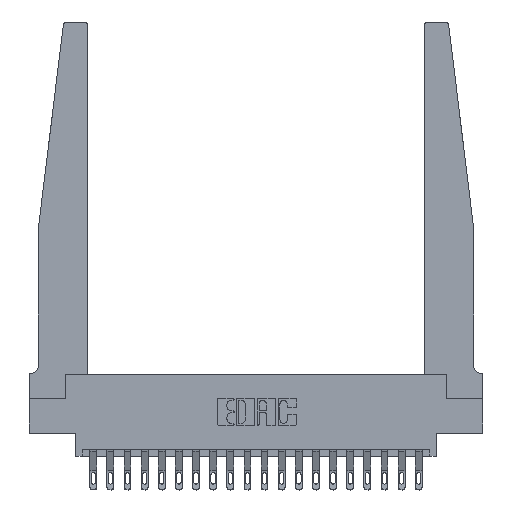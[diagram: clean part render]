
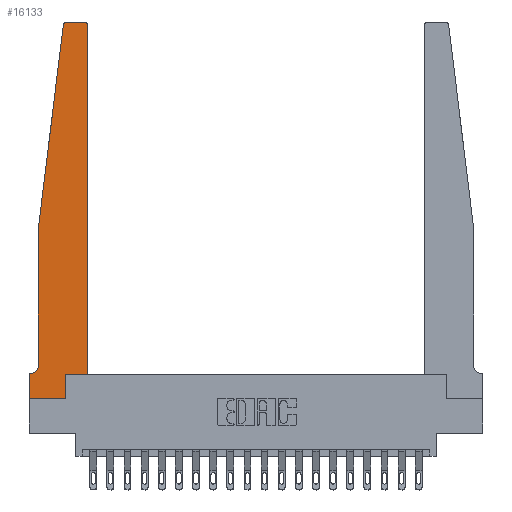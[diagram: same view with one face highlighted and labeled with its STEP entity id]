
A CAD part, top view. The second image highlights one B-rep face of the part: STEP entity #16133.
In plain terms, the highlighted planar face has unit normal (0, 0, 1).
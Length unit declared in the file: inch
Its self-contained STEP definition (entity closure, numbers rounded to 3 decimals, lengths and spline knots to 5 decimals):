
#439 = AXIS2_PLACEMENT_3D ( 'NONE', #8504, #13570, #7630 ) ;
#460 = ORIENTED_EDGE ( 'NONE', *, *, #15996, .T. ) ;
#556 = CARTESIAN_POINT ( 'NONE',  ( 0.425, 0.18, 0.37 ) ) ;
#888 = VERTEX_POINT ( 'NONE', #10330 ) ;
#1077 = DIRECTION ( 'NONE',  ( 0., -1., 0. ) ) ;
#1188 = CARTESIAN_POINT ( 'NONE',  ( 0., 0.1875, 0.37 ) ) ;
#1359 = VECTOR ( 'NONE', #13940, 39.37008 ) ;
#1505 = LINE ( 'NONE', #11701, #17941 ) ;
#1831 = PLANE ( 'NONE',  #439 ) ;
#1939 = DIRECTION ( 'NONE',  ( 1., 0., 0. ) ) ;
#1996 = VERTEX_POINT ( 'NONE', #8567 ) ;
#3223 = AXIS2_PLACEMENT_3D ( 'NONE', #15246, #12058, #15357 ) ;
#3746 = DIRECTION ( 'NONE',  ( 0., 1., 0. ) ) ;
#3941 = EDGE_CURVE ( 'NONE', #10184, #888, #16129, .T. ) ;
#4355 = ORIENTED_EDGE ( 'NONE', *, *, #3941, .T. ) ;
#4744 = LINE ( 'NONE', #11229, #5570 ) ;
#4805 = ORIENTED_EDGE ( 'NONE', *, *, #14903, .T. ) ;
#4994 = CARTESIAN_POINT ( 'NONE',  ( 0.2605, 0.18, 0.37 ) ) ;
#5111 = CARTESIAN_POINT ( 'NONE',  ( 0.065, 1.25, 0.37 ) ) ;
#5184 = EDGE_CURVE ( 'NONE', #16168, #1996, #13847, .T. ) ;
#5434 = CARTESIAN_POINT ( 'NONE',  ( 0.065, 1.25, 0.37 ) ) ;
#5570 = VECTOR ( 'NONE', #6393, 39.37008 ) ;
#5815 = VERTEX_POINT ( 'NONE', #21369 ) ;
#6218 = CARTESIAN_POINT ( 'NONE',  ( 0., 0., 0.37 ) ) ;
#6393 = DIRECTION ( 'NONE',  ( 1., 0., 0. ) ) ;
#6974 = ORIENTED_EDGE ( 'NONE', *, *, #12363, .T. ) ;
#7573 = DIRECTION ( 'NONE',  ( 1., 0., 0. ) ) ;
#7630 = DIRECTION ( 'NONE',  ( 1., 0., 0. ) ) ;
#7911 = LINE ( 'NONE', #16384, #16895 ) ;
#8035 = ORIENTED_EDGE ( 'NONE', *, *, #14879, .T. ) ;
#8504 = CARTESIAN_POINT ( 'NONE',  ( 0., 0.1875, 0.37 ) ) ;
#8559 = VERTEX_POINT ( 'NONE', #21633 ) ;
#8567 = CARTESIAN_POINT ( 'NONE',  ( 0.425, 2.72, 0.37 ) ) ;
#8787 = AXIS2_PLACEMENT_3D ( 'NONE', #10043, #13673, #1939 ) ;
#8823 = DIRECTION ( 'NONE',  ( 0., -1., 0. ) ) ;
#9060 = VECTOR ( 'NONE', #11697, 39.37008 ) ;
#9138 = ORIENTED_EDGE ( 'NONE', *, *, #15578, .T. ) ;
#9245 = VECTOR ( 'NONE', #8823, 39.37008 ) ;
#9516 = DIRECTION ( 'NONE',  ( 0., 0., 1. ) ) ;
#9721 = VERTEX_POINT ( 'NONE', #18452 ) ;
#9821 = LINE ( 'NONE', #5434, #9245 ) ;
#9900 = EDGE_CURVE ( 'NONE', #5815, #16168, #15599, .T. ) ;
#10043 = CARTESIAN_POINT ( 'NONE',  ( 0.27653, 2.72, 0.37 ) ) ;
#10184 = VERTEX_POINT ( 'NONE', #1188 ) ;
#10258 = VECTOR ( 'NONE', #3746, 39.37008 ) ;
#10330 = CARTESIAN_POINT ( 'NONE',  ( 0., 0., 0.37 ) ) ;
#10697 = ORIENTED_EDGE ( 'NONE', *, *, #9900, .T. ) ;
#11091 = ORIENTED_EDGE ( 'NONE', *, *, #12019, .T. ) ;
#11229 = CARTESIAN_POINT ( 'NONE',  ( 0., 0., 0.37 ) ) ;
#11468 = VERTEX_POINT ( 'NONE', #18428 ) ;
#11697 = DIRECTION ( 'NONE',  ( -0.122, -0.992, 0. ) ) ;
#11701 = CARTESIAN_POINT ( 'NONE',  ( 0.065, 0.1875, 0.37 ) ) ;
#11726 = VERTEX_POINT ( 'NONE', #16111 ) ;
#11958 = VECTOR ( 'NONE', #15109, 39.37008 ) ;
#12013 = ORIENTED_EDGE ( 'NONE', *, *, #19616, .T. ) ;
#12019 = EDGE_CURVE ( 'NONE', #18433, #13911, #15321, .T. ) ;
#12058 = DIRECTION ( 'NONE',  ( 0., 0., -1. ) ) ;
#12363 = EDGE_CURVE ( 'NONE', #888, #8559, #4744, .T. ) ;
#12481 = ORIENTED_EDGE ( 'NONE', *, *, #15734, .T. ) ;
#12696 = CARTESIAN_POINT ( 'NONE',  ( 0.24675, 2.72367, 0.37 ) ) ;
#13025 = CIRCLE ( 'NONE', #3223, 0.05 ) ;
#13570 = DIRECTION ( 'NONE',  ( 0., 0., 1. ) ) ;
#13673 = DIRECTION ( 'NONE',  ( 0., 0., 1. ) ) ;
#13790 = AXIS2_PLACEMENT_3D ( 'NONE', #17879, #9516, #7573 ) ;
#13847 = LINE ( 'NONE', #17475, #10258 ) ;
#13911 = VERTEX_POINT ( 'NONE', #14893 ) ;
#13940 = DIRECTION ( 'NONE',  ( 1., 0., 0. ) ) ;
#14299 = DIRECTION ( 'NONE',  ( -1., 0., 0. ) ) ;
#14879 = EDGE_CURVE ( 'NONE', #11468, #18433, #20018, .T. ) ;
#14893 = CARTESIAN_POINT ( 'NONE',  ( 0.065, 1.25, 0.37 ) ) ;
#14903 = EDGE_CURVE ( 'NONE', #8559, #5815, #18076, .T. ) ;
#14952 = DIRECTION ( 'NONE',  ( -1., 0., 0. ) ) ;
#15005 = FACE_OUTER_BOUND ( 'NONE', #18747, .T. ) ;
#15109 = DIRECTION ( 'NONE',  ( 0., 1., 0. ) ) ;
#15246 = CARTESIAN_POINT ( 'NONE',  ( 0.015, 0.2375, 0.37 ) ) ;
#15321 = LINE ( 'NONE', #5111, #9060 ) ;
#15357 = DIRECTION ( 'NONE',  ( -1., 0., 0. ) ) ;
#15578 = EDGE_CURVE ( 'NONE', #11726, #11468, #7911, .T. ) ;
#15599 = LINE ( 'NONE', #556, #1359 ) ;
#15734 = EDGE_CURVE ( 'NONE', #9721, #20816, #13025, .T. ) ;
#15996 = EDGE_CURVE ( 'NONE', #20816, #10184, #1505, .T. ) ;
#16111 = CARTESIAN_POINT ( 'NONE',  ( 0.395, 2.75, 0.37 ) ) ;
#16129 = LINE ( 'NONE', #6218, #20458 ) ;
#16133 = ADVANCED_FACE ( 'NONE', ( #15005 ), #1831, .T. ) ;
#16168 = VERTEX_POINT ( 'NONE', #18847 ) ;
#16384 = CARTESIAN_POINT ( 'NONE',  ( 0.25, 2.75, 0.37 ) ) ;
#16895 = VECTOR ( 'NONE', #14299, 39.37008 ) ;
#17260 = CARTESIAN_POINT ( 'NONE',  ( 0.015, 0.1875, 0.37 ) ) ;
#17316 = CIRCLE ( 'NONE', #13790, 0.03 ) ;
#17475 = CARTESIAN_POINT ( 'NONE',  ( 0.425, 0.18, 0.37 ) ) ;
#17685 = ORIENTED_EDGE ( 'NONE', *, *, #20126, .T. ) ;
#17879 = CARTESIAN_POINT ( 'NONE',  ( 0.395, 2.72, 0.37 ) ) ;
#17941 = VECTOR ( 'NONE', #14952, 39.37008 ) ;
#18076 = LINE ( 'NONE', #4994, #11958 ) ;
#18428 = CARTESIAN_POINT ( 'NONE',  ( 0.27653, 2.75, 0.37 ) ) ;
#18433 = VERTEX_POINT ( 'NONE', #12696 ) ;
#18452 = CARTESIAN_POINT ( 'NONE',  ( 0.065, 0.2375, 0.37 ) ) ;
#18747 = EDGE_LOOP ( 'NONE', ( #9138, #8035, #11091, #17685, #12481, #460, #4355, #6974, #4805, #10697, #20633, #12013 ) ) ;
#18847 = CARTESIAN_POINT ( 'NONE',  ( 0.425, 0.18, 0.37 ) ) ;
#19616 = EDGE_CURVE ( 'NONE', #1996, #11726, #17316, .T. ) ;
#20018 = CIRCLE ( 'NONE', #8787, 0.03 ) ;
#20126 = EDGE_CURVE ( 'NONE', #13911, #9721, #9821, .T. ) ;
#20458 = VECTOR ( 'NONE', #1077, 39.37008 ) ;
#20633 = ORIENTED_EDGE ( 'NONE', *, *, #5184, .T. ) ;
#20816 = VERTEX_POINT ( 'NONE', #17260 ) ;
#21369 = CARTESIAN_POINT ( 'NONE',  ( 0.2605, 0.18, 0.37 ) ) ;
#21633 = CARTESIAN_POINT ( 'NONE',  ( 0.2605, 0., 0.37 ) ) ;
